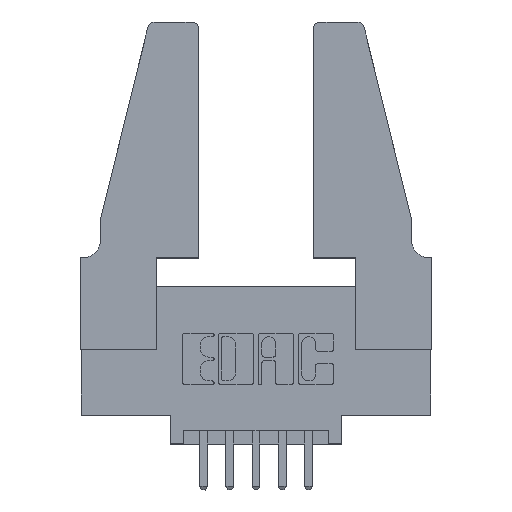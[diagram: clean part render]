
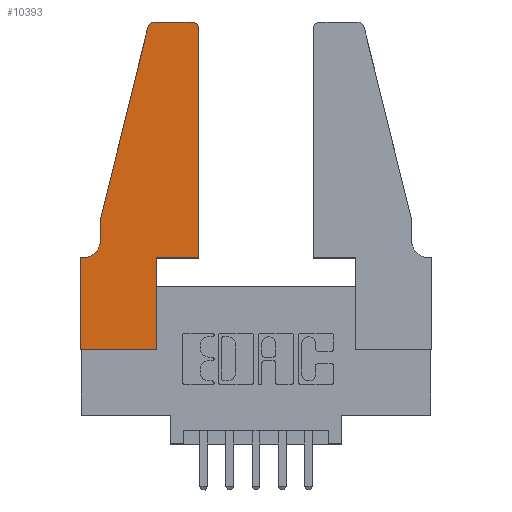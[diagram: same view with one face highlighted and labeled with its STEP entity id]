
A CAD part, top view. The second image highlights one B-rep face of the part: STEP entity #10393.
In plain terms, the highlighted planar face has unit normal (0, 0, 1).
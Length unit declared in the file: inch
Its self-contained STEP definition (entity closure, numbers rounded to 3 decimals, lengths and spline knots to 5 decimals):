
#343 = VERTEX_POINT ( 'NONE', #1358 ) ;
#424 = CIRCLE ( 'NONE', #10926, 0.03 ) ;
#441 = CARTESIAN_POINT ( 'NONE',  ( 0.4505, 1.22, 0.37 ) ) ;
#445 = VERTEX_POINT ( 'NONE', #5654 ) ;
#618 = CARTESIAN_POINT ( 'NONE',  ( 0.0755, 0.5, 0.37 ) ) ;
#622 = LINE ( 'NONE', #4869, #9622 ) ;
#635 = DIRECTION ( 'NONE',  ( 0., 0., -1. ) ) ;
#691 = DIRECTION ( 'NONE',  ( -0.239, -0.971, 0. ) ) ;
#807 = VERTEX_POINT ( 'NONE', #5633 ) ;
#1105 = DIRECTION ( 'NONE',  ( 0., -1., 0. ) ) ;
#1107 = DIRECTION ( 'NONE',  ( 0., -1., 0. ) ) ;
#1167 = CARTESIAN_POINT ( 'NONE',  ( 0., 0., 0.37 ) ) ;
#1177 = LINE ( 'NONE', #11027, #5707 ) ;
#1357 = LINE ( 'NONE', #618, #4917 ) ;
#1358 = CARTESIAN_POINT ( 'NONE',  ( 0.25487, 1.22718, 0.37 ) ) ;
#1362 = CARTESIAN_POINT ( 'NONE',  ( 0., 0.35, 0.37 ) ) ;
#1455 = CARTESIAN_POINT ( 'NONE',  ( 0.4505, 0.35, 0.37 ) ) ;
#1616 = VERTEX_POINT ( 'NONE', #2430 ) ;
#1749 = LINE ( 'NONE', #9513, #10316 ) ;
#1815 = VERTEX_POINT ( 'NONE', #10517 ) ;
#1936 = ORIENTED_EDGE ( 'NONE', *, *, #8700, .T. ) ;
#1945 = EDGE_LOOP ( 'NONE', ( #8144, #10530, #5224, #9909, #2552, #4553, #6558, #1936, #10772, #4977, #7954, #10665 ) ) ;
#2139 = LINE ( 'NONE', #2801, #10455 ) ;
#2142 = FACE_OUTER_BOUND ( 'NONE', #1945, .T. ) ;
#2200 = EDGE_CURVE ( 'NONE', #343, #5235, #1357, .T. ) ;
#2233 = DIRECTION ( 'NONE',  ( 1., 0., 0. ) ) ;
#2253 = CARTESIAN_POINT ( 'NONE',  ( 0.0055, 0.42, 0.37 ) ) ;
#2430 = CARTESIAN_POINT ( 'NONE',  ( 0.4205, 1.25, 0.37 ) ) ;
#2552 = ORIENTED_EDGE ( 'NONE', *, *, #5878, .T. ) ;
#2597 = DIRECTION ( 'NONE',  ( 1., 0., 0. ) ) ;
#2762 = DIRECTION ( 'NONE',  ( 1., 0., 0. ) ) ;
#2801 = CARTESIAN_POINT ( 'NONE',  ( 0., 0., 0.37 ) ) ;
#2814 = AXIS2_PLACEMENT_3D ( 'NONE', #8740, #7959, #2762 ) ;
#3094 = EDGE_CURVE ( 'NONE', #11223, #9202, #10751, .T. ) ;
#3408 = DIRECTION ( 'NONE',  ( 0., 1., 0. ) ) ;
#3512 = VECTOR ( 'NONE', #10795, 39.37008 ) ;
#3812 = VERTEX_POINT ( 'NONE', #8319 ) ;
#3949 = DIRECTION ( 'NONE',  ( 0., 0., 1. ) ) ;
#4310 = CIRCLE ( 'NONE', #2814, 0.03 ) ;
#4553 = ORIENTED_EDGE ( 'NONE', *, *, #4951, .T. ) ;
#4738 = LINE ( 'NONE', #5640, #3512 ) ;
#4837 = DIRECTION ( 'NONE',  ( -1., 0., 0. ) ) ;
#4869 = CARTESIAN_POINT ( 'NONE',  ( 0.0755, 0.35, 0.37 ) ) ;
#4891 = EDGE_CURVE ( 'NONE', #11171, #11223, #1177, .T. ) ;
#4892 = EDGE_CURVE ( 'NONE', #5167, #807, #2139, .T. ) ;
#4917 = VECTOR ( 'NONE', #691, 39.37008 ) ;
#4951 = EDGE_CURVE ( 'NONE', #1815, #5167, #622, .T. ) ;
#4977 = ORIENTED_EDGE ( 'NONE', *, *, #4891, .T. ) ;
#5042 = EDGE_CURVE ( 'NONE', #1616, #11308, #4738, .T. ) ;
#5078 = VECTOR ( 'NONE', #1105, 39.37008 ) ;
#5167 = VERTEX_POINT ( 'NONE', #5781 ) ;
#5224 = ORIENTED_EDGE ( 'NONE', *, *, #2200, .T. ) ;
#5235 = VERTEX_POINT ( 'NONE', #11278 ) ;
#5633 = CARTESIAN_POINT ( 'NONE',  ( 0., 0., 0.37 ) ) ;
#5640 = CARTESIAN_POINT ( 'NONE',  ( 0.2605, 1.25, 0.37 ) ) ;
#5654 = CARTESIAN_POINT ( 'NONE',  ( 0.0755, 0.42, 0.37 ) ) ;
#5707 = VECTOR ( 'NONE', #2233, 39.37008 ) ;
#5781 = CARTESIAN_POINT ( 'NONE',  ( 0., 0.35, 0.37 ) ) ;
#5878 = EDGE_CURVE ( 'NONE', #445, #1815, #7692, .T. ) ;
#6390 = VECTOR ( 'NONE', #11046, 39.37008 ) ;
#6405 = EDGE_CURVE ( 'NONE', #9202, #1616, #4310, .T. ) ;
#6415 = LINE ( 'NONE', #8118, #5078 ) ;
#6416 = AXIS2_PLACEMENT_3D ( 'NONE', #1362, #3949, #7375 ) ;
#6558 = ORIENTED_EDGE ( 'NONE', *, *, #4892, .T. ) ;
#6662 = EDGE_CURVE ( 'NONE', #11308, #343, #424, .T. ) ;
#6816 = CARTESIAN_POINT ( 'NONE',  ( 0.284, 1.22, 0.37 ) ) ;
#7109 = AXIS2_PLACEMENT_3D ( 'NONE', #2253, #635, #11086 ) ;
#7375 = DIRECTION ( 'NONE',  ( 1., 0., 0. ) ) ;
#7692 = CIRCLE ( 'NONE', #7109, 0.07 ) ;
#7954 = ORIENTED_EDGE ( 'NONE', *, *, #3094, .T. ) ;
#7959 = DIRECTION ( 'NONE',  ( 0., 0., 1. ) ) ;
#8118 = CARTESIAN_POINT ( 'NONE',  ( 0.0755, 0.5, 0.37 ) ) ;
#8144 = ORIENTED_EDGE ( 'NONE', *, *, #5042, .T. ) ;
#8173 = PLANE ( 'NONE',  #6416 ) ;
#8286 = EDGE_CURVE ( 'NONE', #5235, #445, #6415, .T. ) ;
#8319 = CARTESIAN_POINT ( 'NONE',  ( 0.2865, 0., 0.37 ) ) ;
#8401 = DIRECTION ( 'NONE',  ( 1., 0., 0. ) ) ;
#8700 = EDGE_CURVE ( 'NONE', #807, #3812, #9651, .T. ) ;
#8740 = CARTESIAN_POINT ( 'NONE',  ( 0.4205, 1.22, 0.37 ) ) ;
#9202 = VERTEX_POINT ( 'NONE', #441 ) ;
#9513 = CARTESIAN_POINT ( 'NONE',  ( 0.2865, 0.35, 0.37 ) ) ;
#9622 = VECTOR ( 'NONE', #4837, 39.37008 ) ;
#9651 = LINE ( 'NONE', #1167, #11311 ) ;
#9909 = ORIENTED_EDGE ( 'NONE', *, *, #8286, .T. ) ;
#9940 = EDGE_CURVE ( 'NONE', #3812, #11171, #1749, .T. ) ;
#10174 = CARTESIAN_POINT ( 'NONE',  ( 0.4505, 0.35, 0.37 ) ) ;
#10316 = VECTOR ( 'NONE', #3408, 39.37008 ) ;
#10332 = DIRECTION ( 'NONE',  ( 0., 0., 1. ) ) ;
#10335 = CARTESIAN_POINT ( 'NONE',  ( 0.2865, 0.35, 0.37 ) ) ;
#10393 = ADVANCED_FACE ( 'NONE', ( #2142 ), #8173, .T. ) ;
#10455 = VECTOR ( 'NONE', #1107, 39.37008 ) ;
#10479 = CARTESIAN_POINT ( 'NONE',  ( 0.284, 1.25, 0.37 ) ) ;
#10517 = CARTESIAN_POINT ( 'NONE',  ( 0.0055, 0.35, 0.37 ) ) ;
#10530 = ORIENTED_EDGE ( 'NONE', *, *, #6662, .T. ) ;
#10665 = ORIENTED_EDGE ( 'NONE', *, *, #6405, .T. ) ;
#10751 = LINE ( 'NONE', #10174, #6390 ) ;
#10772 = ORIENTED_EDGE ( 'NONE', *, *, #9940, .T. ) ;
#10795 = DIRECTION ( 'NONE',  ( -1., 0., 0. ) ) ;
#10926 = AXIS2_PLACEMENT_3D ( 'NONE', #6816, #10332, #2597 ) ;
#11027 = CARTESIAN_POINT ( 'NONE',  ( 0.4505, 0.35, 0.37 ) ) ;
#11046 = DIRECTION ( 'NONE',  ( 0., 1., 0. ) ) ;
#11086 = DIRECTION ( 'NONE',  ( -1., 0., 0. ) ) ;
#11171 = VERTEX_POINT ( 'NONE', #10335 ) ;
#11223 = VERTEX_POINT ( 'NONE', #1455 ) ;
#11278 = CARTESIAN_POINT ( 'NONE',  ( 0.0755, 0.5, 0.37 ) ) ;
#11308 = VERTEX_POINT ( 'NONE', #10479 ) ;
#11311 = VECTOR ( 'NONE', #8401, 39.37008 ) ;
